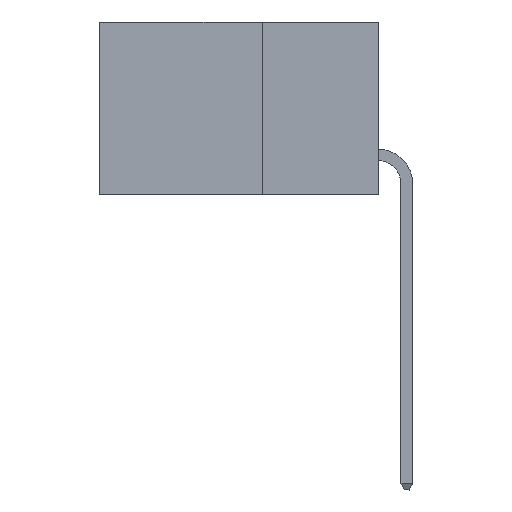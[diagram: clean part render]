
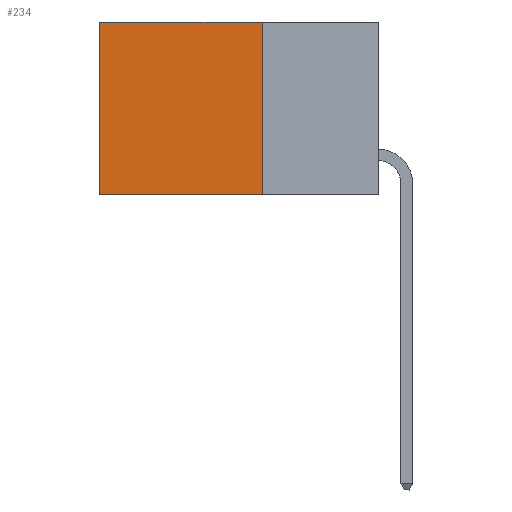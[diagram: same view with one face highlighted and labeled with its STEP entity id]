
A CAD part, left-side view. The second image highlights one B-rep face of the part: STEP entity #234.
In plain terms, the highlighted planar face has unit normal (-1, 0, 0).
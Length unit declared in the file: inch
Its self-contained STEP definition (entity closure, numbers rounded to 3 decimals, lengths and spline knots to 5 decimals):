
#234 = ADVANCED_FACE ( 'NONE', ( #6635 ), #15120, .F. ) ;
#2252 = VERTEX_POINT ( 'NONE', #8364 ) ;
#2850 = VERTEX_POINT ( 'NONE', #9839 ) ;
#3295 = CARTESIAN_POINT ( 'NONE',  ( 0.298, 0.25, -0.37 ) ) ;
#3692 = CARTESIAN_POINT ( 'NONE',  ( 0.298, 0.6, 0. ) ) ;
#3812 = DIRECTION ( 'NONE',  ( 0., 0., -1. ) ) ;
#3994 = ORIENTED_EDGE ( 'NONE', *, *, #10001, .F. ) ;
#4315 = ORIENTED_EDGE ( 'NONE', *, *, #14047, .F. ) ;
#6635 = FACE_OUTER_BOUND ( 'NONE', #12527, .T. ) ;
#7073 = VECTOR ( 'NONE', #3812, 39.37008 ) ;
#7881 = CARTESIAN_POINT ( 'NONE',  ( 0.298, 0.6, 0. ) ) ;
#8341 = DIRECTION ( 'NONE',  ( 1., 0., 0. ) ) ;
#8364 = CARTESIAN_POINT ( 'NONE',  ( 0.298, 0.25, 0. ) ) ;
#9194 = EDGE_CURVE ( 'NONE', #2252, #15547, #14837, .T. ) ;
#9821 = VECTOR ( 'NONE', #21283, 39.37008 ) ;
#9839 = CARTESIAN_POINT ( 'NONE',  ( 0.298, 0.6, -0.37 ) ) ;
#10001 = EDGE_CURVE ( 'NONE', #2252, #23630, #18832, .T. ) ;
#10483 = DIRECTION ( 'NONE',  ( 0., 0., -1. ) ) ;
#10822 = CARTESIAN_POINT ( 'NONE',  ( 0.298, 0.25, 0. ) ) ;
#10977 = EDGE_CURVE ( 'NONE', #15547, #2850, #13405, .T. ) ;
#12527 = EDGE_LOOP ( 'NONE', ( #19192, #4315, #3994, #20724 ) ) ;
#13405 = LINE ( 'NONE', #3692, #7073 ) ;
#14047 = EDGE_CURVE ( 'NONE', #23630, #2850, #15939, .T. ) ;
#14837 = LINE ( 'NONE', #21359, #9821 ) ;
#15120 = PLANE ( 'NONE',  #25478 ) ;
#15547 = VERTEX_POINT ( 'NONE', #7881 ) ;
#15939 = LINE ( 'NONE', #17951, #25742 ) ;
#17951 = CARTESIAN_POINT ( 'NONE',  ( 0.298, 0.25, -0.37 ) ) ;
#18832 = LINE ( 'NONE', #10822, #23358 ) ;
#19192 = ORIENTED_EDGE ( 'NONE', *, *, #10977, .T. ) ;
#19910 = DIRECTION ( 'NONE',  ( 0., 0., -1. ) ) ;
#20724 = ORIENTED_EDGE ( 'NONE', *, *, #9194, .T. ) ;
#21031 = CARTESIAN_POINT ( 'NONE',  ( 0.298, 0.25, 0. ) ) ;
#21283 = DIRECTION ( 'NONE',  ( 0., 1., 0. ) ) ;
#21359 = CARTESIAN_POINT ( 'NONE',  ( 0.298, 0.25, 0. ) ) ;
#23358 = VECTOR ( 'NONE', #10483, 39.37008 ) ;
#23630 = VERTEX_POINT ( 'NONE', #3295 ) ;
#25043 = DIRECTION ( 'NONE',  ( 0., 1., 0. ) ) ;
#25478 = AXIS2_PLACEMENT_3D ( 'NONE', #21031, #8341, #19910 ) ;
#25742 = VECTOR ( 'NONE', #25043, 39.37008 ) ;
